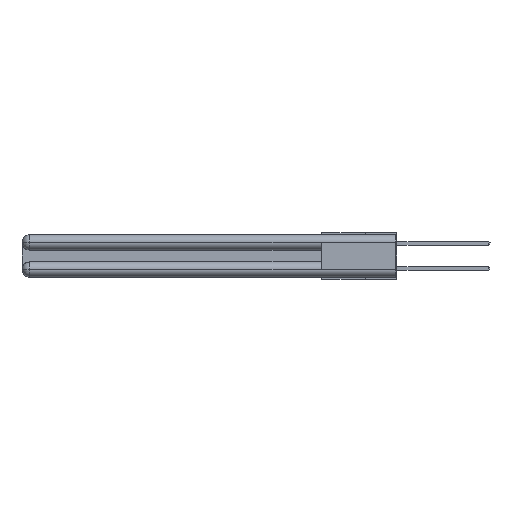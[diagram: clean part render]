
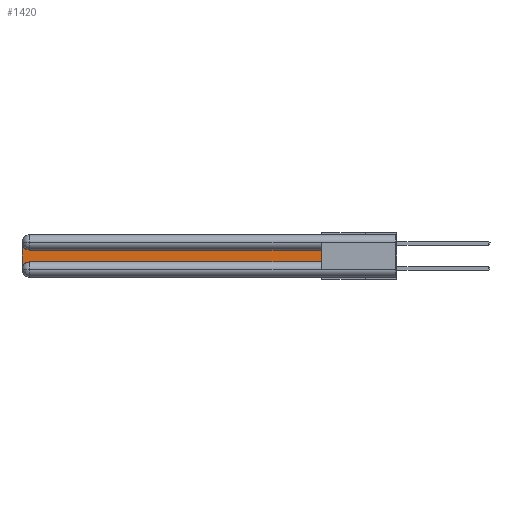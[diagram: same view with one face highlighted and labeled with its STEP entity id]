
A CAD part, left-side view. The second image highlights one B-rep face of the part: STEP entity #1420.
In plain terms, the highlighted planar face has unit normal (-1, 0, 0).
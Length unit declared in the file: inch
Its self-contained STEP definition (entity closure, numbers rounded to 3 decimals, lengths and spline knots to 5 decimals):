
#257 = EDGE_CURVE ( 'NONE', #26823, #30387, #13879, .T. ) ;
#280 = VERTEX_POINT ( 'NONE', #6406 ) ;
#374 = EDGE_CURVE ( 'NONE', #30387, #14433, #26288, .T. ) ;
#441 = DIRECTION ( 'NONE',  ( 0., 0., -1. ) ) ;
#1104 = DIRECTION ( 'NONE',  ( 1., 0., 0. ) ) ;
#1336 = LINE ( 'NONE', #5450, #13686 ) ;
#1420 = ADVANCED_FACE ( 'NONE', ( #10751 ), #14196, .F. ) ;
#2679 = VECTOR ( 'NONE', #9201, 39.37008 ) ;
#2819 = ORIENTED_EDGE ( 'NONE', *, *, #29278, .T. ) ;
#4460 = EDGE_LOOP ( 'NONE', ( #2819, #5412, #7542, #26820, #12174, #31463 ) ) ;
#5199 = CARTESIAN_POINT ( 'NONE',  ( 0.075, 2.94, -0.2775 ) ) ;
#5412 = ORIENTED_EDGE ( 'NONE', *, *, #7662, .T. ) ;
#5440 = CARTESIAN_POINT ( 'NONE',  ( 0.075, 0.6, -0.2175 ) ) ;
#5450 = CARTESIAN_POINT ( 'NONE',  ( 0.075, 0.6, -0.1225 ) ) ;
#6406 = CARTESIAN_POINT ( 'NONE',  ( 0.075, 0.6, -0.1225 ) ) ;
#7542 = ORIENTED_EDGE ( 'NONE', *, *, #257, .T. ) ;
#7662 = EDGE_CURVE ( 'NONE', #18710, #26823, #22148, .T. ) ;
#8385 = CARTESIAN_POINT ( 'NONE',  ( 0.075, 3., -0.2175 ) ) ;
#9201 = DIRECTION ( 'NONE',  ( 0., 0., -1. ) ) ;
#10154 = CARTESIAN_POINT ( 'NONE',  ( 0.075, 0.6, -0.2175 ) ) ;
#10751 = FACE_OUTER_BOUND ( 'NONE', #4460, .T. ) ;
#11961 = DIRECTION ( 'NONE',  ( 1., 0., 0. ) ) ;
#12020 = AXIS2_PLACEMENT_3D ( 'NONE', #21753, #11961, #16889 ) ;
#12174 = ORIENTED_EDGE ( 'NONE', *, *, #25775, .T. ) ;
#12210 = AXIS2_PLACEMENT_3D ( 'NONE', #5199, #25113, #441 ) ;
#12422 = CARTESIAN_POINT ( 'NONE',  ( 0.075, 3., -0.0625 ) ) ;
#12564 = DIRECTION ( 'NONE',  ( 0., 0., 1. ) ) ;
#12929 = CARTESIAN_POINT ( 'NONE',  ( 0.075, 2.94, -0.2175 ) ) ;
#13686 = VECTOR ( 'NONE', #25480, 39.37008 ) ;
#13879 = LINE ( 'NONE', #8385, #2679 ) ;
#14196 = PLANE ( 'NONE',  #12020 ) ;
#14433 = VERTEX_POINT ( 'NONE', #12929 ) ;
#14835 = CARTESIAN_POINT ( 'NONE',  ( 0.075, 2.94, -0.1225 ) ) ;
#16601 = CARTESIAN_POINT ( 'NONE',  ( 0.075, 3., -0.2775 ) ) ;
#16889 = DIRECTION ( 'NONE',  ( 0., 0., -1. ) ) ;
#18364 = DIRECTION ( 'NONE',  ( 0., 0., -1. ) ) ;
#18710 = VERTEX_POINT ( 'NONE', #14835 ) ;
#20165 = VECTOR ( 'NONE', #27471, 39.37008 ) ;
#21753 = CARTESIAN_POINT ( 'NONE',  ( 0.075, 3., -0.1225 ) ) ;
#22148 = CIRCLE ( 'NONE', #25643, 0.06 ) ;
#22617 = CARTESIAN_POINT ( 'NONE',  ( 0.075, 0.6, -0.2175 ) ) ;
#22867 = LINE ( 'NONE', #10154, #20165 ) ;
#23809 = VERTEX_POINT ( 'NONE', #22617 ) ;
#25113 = DIRECTION ( 'NONE',  ( 1., 0., 0. ) ) ;
#25480 = DIRECTION ( 'NONE',  ( 0., 1., 0. ) ) ;
#25643 = AXIS2_PLACEMENT_3D ( 'NONE', #28339, #1104, #18364 ) ;
#25775 = EDGE_CURVE ( 'NONE', #14433, #23809, #22867, .T. ) ;
#26288 = CIRCLE ( 'NONE', #12210, 0.06 ) ;
#26820 = ORIENTED_EDGE ( 'NONE', *, *, #374, .T. ) ;
#26823 = VERTEX_POINT ( 'NONE', #12422 ) ;
#27471 = DIRECTION ( 'NONE',  ( 0., -1., 0. ) ) ;
#27493 = LINE ( 'NONE', #5440, #28275 ) ;
#28275 = VECTOR ( 'NONE', #12564, 39.37008 ) ;
#28339 = CARTESIAN_POINT ( 'NONE',  ( 0.075, 2.94, -0.0625 ) ) ;
#29278 = EDGE_CURVE ( 'NONE', #280, #18710, #1336, .T. ) ;
#30387 = VERTEX_POINT ( 'NONE', #16601 ) ;
#31409 = EDGE_CURVE ( 'NONE', #23809, #280, #27493, .T. ) ;
#31463 = ORIENTED_EDGE ( 'NONE', *, *, #31409, .T. ) ;
